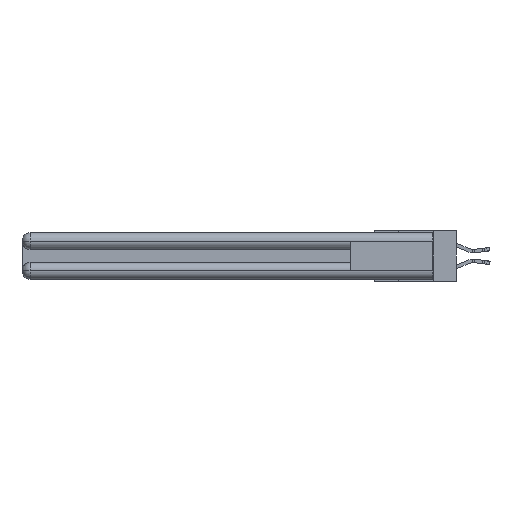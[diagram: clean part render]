
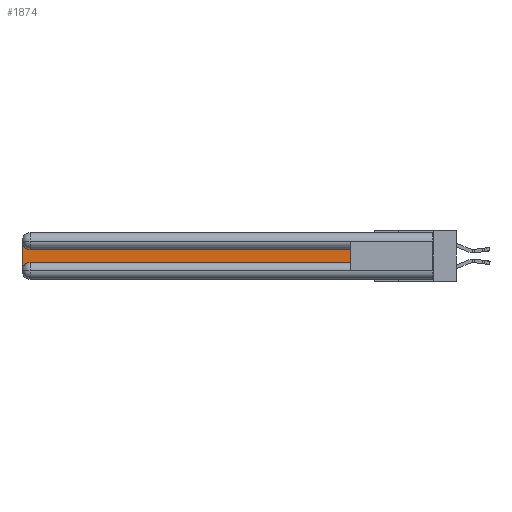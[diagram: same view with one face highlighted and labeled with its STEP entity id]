
A CAD part, left-side view. The second image highlights one B-rep face of the part: STEP entity #1874.
In plain terms, the highlighted planar face has unit normal (-1, 0, 0).
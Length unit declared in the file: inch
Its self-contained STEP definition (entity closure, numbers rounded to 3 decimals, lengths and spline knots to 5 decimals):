
#95 = VECTOR ( 'NONE', #13483, 39.37008 ) ;
#347 = DIRECTION ( 'NONE',  ( 0., 0., -1. ) ) ;
#354 = VECTOR ( 'NONE', #32357, 39.37008 ) ;
#527 = ORIENTED_EDGE ( 'NONE', *, *, #23876, .T. ) ;
#1624 = EDGE_CURVE ( 'NONE', #20170, #22341, #25484, .T. ) ;
#1874 = ADVANCED_FACE ( 'NONE', ( #23491 ), #4834, .F. ) ;
#1896 = DIRECTION ( 'NONE',  ( 1., 0., 0. ) ) ;
#2565 = CARTESIAN_POINT ( 'NONE',  ( 0.075, 3., -0.2775 ) ) ;
#3973 = ORIENTED_EDGE ( 'NONE', *, *, #24678, .T. ) ;
#4278 = VERTEX_POINT ( 'NONE', #29775 ) ;
#4834 = PLANE ( 'NONE',  #8148 ) ;
#6200 = CIRCLE ( 'NONE', #29707, 0.06 ) ;
#7424 = CARTESIAN_POINT ( 'NONE',  ( 0.075, 3., -0.1225 ) ) ;
#7743 = DIRECTION ( 'NONE',  ( 1., 0., 0. ) ) ;
#8089 = CARTESIAN_POINT ( 'NONE',  ( 0.075, 3., -0.2175 ) ) ;
#8148 = AXIS2_PLACEMENT_3D ( 'NONE', #7424, #14601, #15047 ) ;
#8403 = ORIENTED_EDGE ( 'NONE', *, *, #18124, .T. ) ;
#9445 = VERTEX_POINT ( 'NONE', #21703 ) ;
#11440 = CARTESIAN_POINT ( 'NONE',  ( 0.075, 2.94, -0.1225 ) ) ;
#12124 = VECTOR ( 'NONE', #347, 39.37008 ) ;
#13483 = DIRECTION ( 'NONE',  ( 0., 1., 0. ) ) ;
#13689 = EDGE_LOOP ( 'NONE', ( #3973, #8403, #20268, #25273, #527, #15580 ) ) ;
#14601 = DIRECTION ( 'NONE',  ( 1., 0., 0. ) ) ;
#15047 = DIRECTION ( 'NONE',  ( 0., 0., -1. ) ) ;
#15580 = ORIENTED_EDGE ( 'NONE', *, *, #1624, .T. ) ;
#16707 = DIRECTION ( 'NONE',  ( 0., 0., -1. ) ) ;
#16719 = CARTESIAN_POINT ( 'NONE',  ( 0.075, 0.6, -0.2175 ) ) ;
#17174 = CARTESIAN_POINT ( 'NONE',  ( 0.075, 0.6, -0.2175 ) ) ;
#18124 = EDGE_CURVE ( 'NONE', #23532, #4278, #6200, .T. ) ;
#19577 = LINE ( 'NONE', #8089, #12124 ) ;
#20170 = VERTEX_POINT ( 'NONE', #16719 ) ;
#20268 = ORIENTED_EDGE ( 'NONE', *, *, #30048, .T. ) ;
#20860 = AXIS2_PLACEMENT_3D ( 'NONE', #22810, #7743, #25346 ) ;
#21703 = CARTESIAN_POINT ( 'NONE',  ( 0.075, 2.94, -0.2175 ) ) ;
#21787 = VERTEX_POINT ( 'NONE', #2565 ) ;
#22341 = VERTEX_POINT ( 'NONE', #28700 ) ;
#22810 = CARTESIAN_POINT ( 'NONE',  ( 0.075, 2.94, -0.2775 ) ) ;
#22834 = CARTESIAN_POINT ( 'NONE',  ( 0.075, 0.6, -0.2175 ) ) ;
#23491 = FACE_OUTER_BOUND ( 'NONE', #13689, .T. ) ;
#23532 = VERTEX_POINT ( 'NONE', #11440 ) ;
#23876 = EDGE_CURVE ( 'NONE', #9445, #20170, #25650, .T. ) ;
#24383 = CARTESIAN_POINT ( 'NONE',  ( 0.075, 2.94, -0.0625 ) ) ;
#24433 = LINE ( 'NONE', #28154, #95 ) ;
#24678 = EDGE_CURVE ( 'NONE', #22341, #23532, #24433, .T. ) ;
#25273 = ORIENTED_EDGE ( 'NONE', *, *, #27192, .T. ) ;
#25284 = VECTOR ( 'NONE', #25482, 39.37008 ) ;
#25346 = DIRECTION ( 'NONE',  ( 0., 0., -1. ) ) ;
#25482 = DIRECTION ( 'NONE',  ( 0., -1., 0. ) ) ;
#25484 = LINE ( 'NONE', #17174, #354 ) ;
#25650 = LINE ( 'NONE', #22834, #25284 ) ;
#27192 = EDGE_CURVE ( 'NONE', #21787, #9445, #31493, .T. ) ;
#28154 = CARTESIAN_POINT ( 'NONE',  ( 0.075, 0.6, -0.1225 ) ) ;
#28700 = CARTESIAN_POINT ( 'NONE',  ( 0.075, 0.6, -0.1225 ) ) ;
#29707 = AXIS2_PLACEMENT_3D ( 'NONE', #24383, #1896, #16707 ) ;
#29775 = CARTESIAN_POINT ( 'NONE',  ( 0.075, 3., -0.0625 ) ) ;
#30048 = EDGE_CURVE ( 'NONE', #4278, #21787, #19577, .T. ) ;
#31493 = CIRCLE ( 'NONE', #20860, 0.06 ) ;
#32357 = DIRECTION ( 'NONE',  ( 0., 0., 1. ) ) ;
